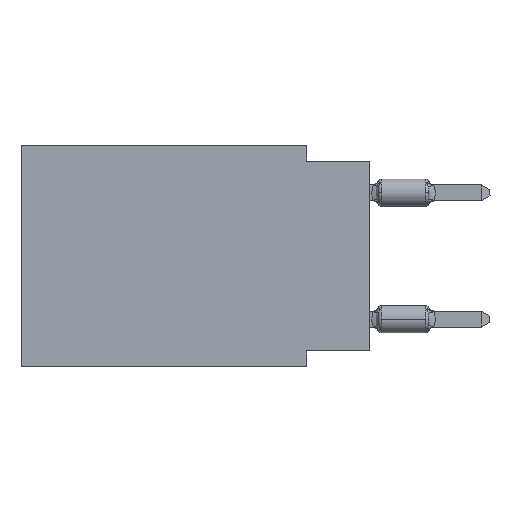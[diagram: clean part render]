
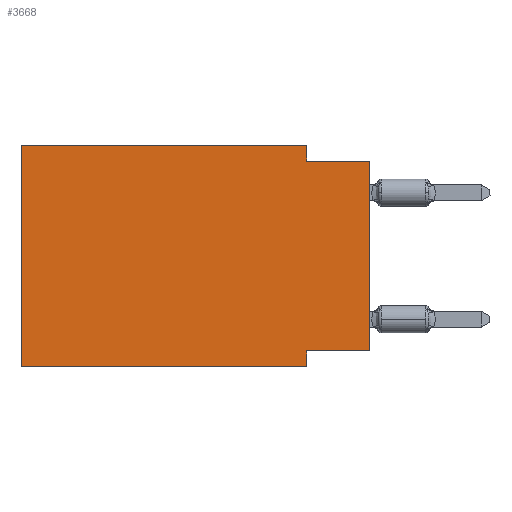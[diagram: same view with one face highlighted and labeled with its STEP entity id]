
A CAD part, left-side view. The second image highlights one B-rep face of the part: STEP entity #3668.
In plain terms, the highlighted planar face has unit normal (-1, 0, 0).
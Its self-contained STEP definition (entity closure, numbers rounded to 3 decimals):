
#284 = CARTESIAN_POINT ( 'NONE',  ( 0., 0., -0.635 ) ) ;
#459 = VECTOR ( 'NONE', #2692, 1000. ) ;
#893 = CARTESIAN_POINT ( 'NONE',  ( 0., 0., -8.255 ) ) ;
#1041 = DIRECTION ( 'NONE',  ( 0., -1., 0. ) ) ;
#1122 = VERTEX_POINT ( 'NONE', #13040 ) ;
#1273 = LINE ( 'NONE', #3534, #8165 ) ;
#1361 = CARTESIAN_POINT ( 'NONE',  ( 0., 13.97, 0. ) ) ;
#1374 = CARTESIAN_POINT ( 'NONE',  ( 0., 2.54, -8.255 ) ) ;
#1580 = FACE_OUTER_BOUND ( 'NONE', #14924, .T. ) ;
#1749 = VERTEX_POINT ( 'NONE', #8895 ) ;
#2177 = LINE ( 'NONE', #893, #12511 ) ;
#2329 = CARTESIAN_POINT ( 'NONE',  ( 0., 2.54, -8.89 ) ) ;
#2402 = LINE ( 'NONE', #12937, #6654 ) ;
#2686 = ORIENTED_EDGE ( 'NONE', *, *, #10686, .T. ) ;
#2692 = DIRECTION ( 'NONE',  ( 0., -1., 0. ) ) ;
#2746 = AXIS2_PLACEMENT_3D ( 'NONE', #14478, #11967, #8705 ) ;
#3396 = DIRECTION ( 'NONE',  ( 0., 0., -1. ) ) ;
#3534 = CARTESIAN_POINT ( 'NONE',  ( 0., 13.97, 0. ) ) ;
#3627 = DIRECTION ( 'NONE',  ( 0., 0., 1. ) ) ;
#3668 = ADVANCED_FACE ( 'NONE', ( #1580 ), #6124, .F. ) ;
#3831 = ORIENTED_EDGE ( 'NONE', *, *, #7860, .F. ) ;
#4233 = LINE ( 'NONE', #8862, #5022 ) ;
#4673 = LINE ( 'NONE', #2329, #7915 ) ;
#4737 = DIRECTION ( 'NONE',  ( 0., 0., -1. ) ) ;
#5022 = VECTOR ( 'NONE', #14793, 1000. ) ;
#5205 = VERTEX_POINT ( 'NONE', #5968 ) ;
#5314 = ORIENTED_EDGE ( 'NONE', *, *, #14173, .F. ) ;
#5590 = EDGE_CURVE ( 'NONE', #13044, #10436, #2177, .T. ) ;
#5968 = CARTESIAN_POINT ( 'NONE',  ( 0., 2.54, -8.89 ) ) ;
#6124 = PLANE ( 'NONE',  #2746 ) ;
#6446 = ORIENTED_EDGE ( 'NONE', *, *, #8279, .T. ) ;
#6654 = VECTOR ( 'NONE', #4737, 1000. ) ;
#6850 = CARTESIAN_POINT ( 'NONE',  ( 0., 13.97, -8.89 ) ) ;
#6861 = EDGE_CURVE ( 'NONE', #7202, #1122, #2402, .T. ) ;
#6889 = VECTOR ( 'NONE', #3627, 1000. ) ;
#6941 = DIRECTION ( 'NONE',  ( 0., -1., 0. ) ) ;
#7038 = ORIENTED_EDGE ( 'NONE', *, *, #11711, .F. ) ;
#7202 = VERTEX_POINT ( 'NONE', #11347 ) ;
#7860 = EDGE_CURVE ( 'NONE', #10436, #5205, #4673, .T. ) ;
#7915 = VECTOR ( 'NONE', #3396, 1000. ) ;
#7919 = EDGE_CURVE ( 'NONE', #1749, #7202, #1273, .T. ) ;
#7935 = DIRECTION ( 'NONE',  ( 0., 1., 0. ) ) ;
#8165 = VECTOR ( 'NONE', #6941, 1000. ) ;
#8256 = CARTESIAN_POINT ( 'NONE',  ( 0., 0., -8.255 ) ) ;
#8279 = EDGE_CURVE ( 'NONE', #14092, #5205, #14838, .T. ) ;
#8705 = DIRECTION ( 'NONE',  ( 0., 0., -1. ) ) ;
#8862 = CARTESIAN_POINT ( 'NONE',  ( 0., 0., 0. ) ) ;
#8895 = CARTESIAN_POINT ( 'NONE',  ( 0., 13.97, 0. ) ) ;
#10234 = CARTESIAN_POINT ( 'NONE',  ( 0., 13.97, -8.89 ) ) ;
#10282 = ORIENTED_EDGE ( 'NONE', *, *, #6861, .F. ) ;
#10369 = CARTESIAN_POINT ( 'NONE',  ( 0., 0., -0.635 ) ) ;
#10436 = VERTEX_POINT ( 'NONE', #1374 ) ;
#10669 = LINE ( 'NONE', #284, #459 ) ;
#10686 = EDGE_CURVE ( 'NONE', #13044, #14502, #4233, .T. ) ;
#11347 = CARTESIAN_POINT ( 'NONE',  ( 0., 2.54, 0. ) ) ;
#11443 = ORIENTED_EDGE ( 'NONE', *, *, #7919, .F. ) ;
#11711 = EDGE_CURVE ( 'NONE', #1122, #14502, #10669, .T. ) ;
#11967 = DIRECTION ( 'NONE',  ( 1., 0., 0. ) ) ;
#12277 = VECTOR ( 'NONE', #1041, 1000. ) ;
#12511 = VECTOR ( 'NONE', #7935, 1000. ) ;
#12937 = CARTESIAN_POINT ( 'NONE',  ( 0., 2.54, 0. ) ) ;
#13040 = CARTESIAN_POINT ( 'NONE',  ( 0., 2.54, -0.635 ) ) ;
#13044 = VERTEX_POINT ( 'NONE', #8256 ) ;
#13482 = ORIENTED_EDGE ( 'NONE', *, *, #5590, .F. ) ;
#13721 = LINE ( 'NONE', #1361, #6889 ) ;
#14092 = VERTEX_POINT ( 'NONE', #10234 ) ;
#14173 = EDGE_CURVE ( 'NONE', #14092, #1749, #13721, .T. ) ;
#14478 = CARTESIAN_POINT ( 'NONE',  ( 0., 13.97, 0. ) ) ;
#14502 = VERTEX_POINT ( 'NONE', #10369 ) ;
#14793 = DIRECTION ( 'NONE',  ( 0., 0., 1. ) ) ;
#14838 = LINE ( 'NONE', #6850, #12277 ) ;
#14924 = EDGE_LOOP ( 'NONE', ( #2686, #7038, #10282, #11443, #5314, #6446, #3831, #13482 ) ) ;
